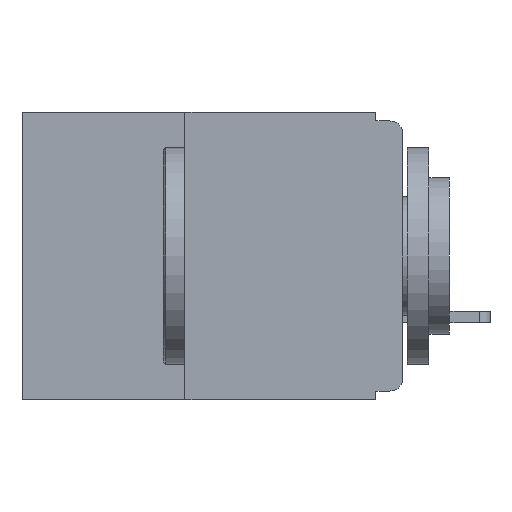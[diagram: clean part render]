
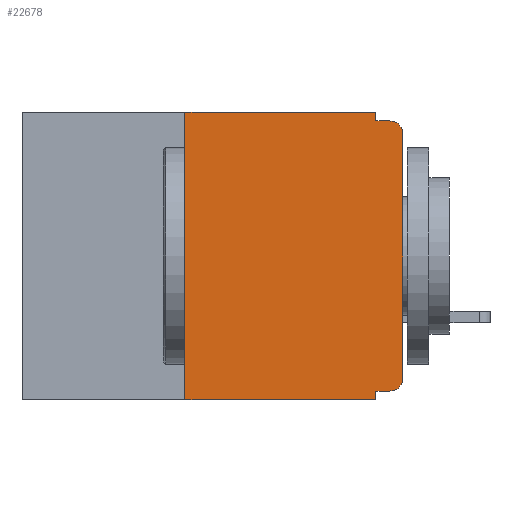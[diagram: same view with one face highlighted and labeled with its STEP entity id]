
A CAD part, left-side view. The second image highlights one B-rep face of the part: STEP entity #22678.
In plain terms, the highlighted planar face has unit normal (-1, 0, 0).
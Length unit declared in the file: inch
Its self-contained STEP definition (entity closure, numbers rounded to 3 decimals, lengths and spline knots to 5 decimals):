
#242 = VECTOR ( 'NONE', #19861, 39.37008 ) ;
#512 = VECTOR ( 'NONE', #14025, 39.37008 ) ;
#592 = CARTESIAN_POINT ( 'NONE',  ( 0., 0.25, -0.33 ) ) ;
#633 = DIRECTION ( 'NONE',  ( 0., 1., 0. ) ) ;
#688 = CARTESIAN_POINT ( 'NONE',  ( 0., 0., -0.305 ) ) ;
#809 = VERTEX_POINT ( 'NONE', #9481 ) ;
#838 = VERTEX_POINT ( 'NONE', #23414 ) ;
#1155 = DIRECTION ( 'NONE',  ( 0., 0., -1. ) ) ;
#1160 = CARTESIAN_POINT ( 'NONE',  ( 0., 0.031, -0.33 ) ) ;
#1646 = LINE ( 'NONE', #13008, #24526 ) ;
#2704 = CIRCLE ( 'NONE', #27872, 0.015 ) ;
#2880 = VECTOR ( 'NONE', #15317, 39.37008 ) ;
#3051 = DIRECTION ( 'NONE',  ( 0., 0., 1. ) ) ;
#3053 = EDGE_CURVE ( 'NONE', #838, #6656, #2704, .T. ) ;
#3118 = VECTOR ( 'NONE', #28104, 39.37008 ) ;
#3181 = ORIENTED_EDGE ( 'NONE', *, *, #4889, .F. ) ;
#4009 = EDGE_CURVE ( 'NONE', #23971, #8865, #12394, .T. ) ;
#4889 = EDGE_CURVE ( 'NONE', #809, #14808, #24730, .T. ) ;
#5514 = LINE ( 'NONE', #11851, #10742 ) ;
#5854 = AXIS2_PLACEMENT_3D ( 'NONE', #21785, #8538, #23991 ) ;
#6191 = ORIENTED_EDGE ( 'NONE', *, *, #4009, .F. ) ;
#6656 = VERTEX_POINT ( 'NONE', #688 ) ;
#7513 = EDGE_CURVE ( 'NONE', #24292, #8865, #10540, .T. ) ;
#7899 = VERTEX_POINT ( 'NONE', #18777 ) ;
#7981 = CARTESIAN_POINT ( 'NONE',  ( 0., 0., -0.025 ) ) ;
#8538 = DIRECTION ( 'NONE',  ( -1., 0., 0. ) ) ;
#8789 = LINE ( 'NONE', #28398, #2880 ) ;
#8865 = VERTEX_POINT ( 'NONE', #26378 ) ;
#9366 = EDGE_CURVE ( 'NONE', #12148, #14808, #26597, .T. ) ;
#9481 = CARTESIAN_POINT ( 'NONE',  ( 0., 0.031, -0.32 ) ) ;
#10540 = CIRCLE ( 'NONE', #5854, 0.015 ) ;
#10575 = CARTESIAN_POINT ( 'NONE',  ( 0., 0.437, -0.33 ) ) ;
#10742 = VECTOR ( 'NONE', #633, 39.37008 ) ;
#10921 = CARTESIAN_POINT ( 'NONE',  ( 0., 0.031, -0.01 ) ) ;
#11686 = PLANE ( 'NONE',  #23596 ) ;
#11851 = CARTESIAN_POINT ( 'NONE',  ( 0., 0., -0.32 ) ) ;
#12148 = VERTEX_POINT ( 'NONE', #592 ) ;
#12394 = LINE ( 'NONE', #13994, #512 ) ;
#13008 = CARTESIAN_POINT ( 'NONE',  ( 0., 0.25, -0.33 ) ) ;
#13031 = VECTOR ( 'NONE', #1155, 39.37008 ) ;
#13483 = EDGE_CURVE ( 'NONE', #838, #809, #5514, .T. ) ;
#13826 = EDGE_CURVE ( 'NONE', #12148, #7899, #1646, .T. ) ;
#13915 = DIRECTION ( 'NONE',  ( 0., 0., -1. ) ) ;
#13994 = CARTESIAN_POINT ( 'NONE',  ( 0., 0., -0.01 ) ) ;
#14025 = DIRECTION ( 'NONE',  ( 0., -1., 0. ) ) ;
#14808 = VERTEX_POINT ( 'NONE', #23632 ) ;
#15317 = DIRECTION ( 'NONE',  ( 0., 0., -1. ) ) ;
#15421 = LINE ( 'NONE', #16335, #16813 ) ;
#15725 = ORIENTED_EDGE ( 'NONE', *, *, #13483, .F. ) ;
#15883 = EDGE_CURVE ( 'NONE', #6656, #24292, #15421, .T. ) ;
#16335 = CARTESIAN_POINT ( 'NONE',  ( 0., 0., 0. ) ) ;
#16719 = FACE_OUTER_BOUND ( 'NONE', #17098, .T. ) ;
#16774 = EDGE_CURVE ( 'NONE', #25740, #23971, #8789, .T. ) ;
#16813 = VECTOR ( 'NONE', #3051, 39.37008 ) ;
#17098 = EDGE_LOOP ( 'NONE', ( #27651, #26703, #6191, #23794, #27467, #21826, #18689, #3181, #15725, #24739 ) ) ;
#18689 = ORIENTED_EDGE ( 'NONE', *, *, #9366, .T. ) ;
#18777 = CARTESIAN_POINT ( 'NONE',  ( 0., 0.25, 0. ) ) ;
#19635 = CARTESIAN_POINT ( 'NONE',  ( 0., 0.031, 0. ) ) ;
#19861 = DIRECTION ( 'NONE',  ( 0., -1., 0. ) ) ;
#21781 = DIRECTION ( 'NONE',  ( 0., 0., 1. ) ) ;
#21785 = CARTESIAN_POINT ( 'NONE',  ( 0., 0.015, -0.025 ) ) ;
#21826 = ORIENTED_EDGE ( 'NONE', *, *, #13826, .F. ) ;
#22678 = ADVANCED_FACE ( 'NONE', ( #16719 ), #11686, .F. ) ;
#23414 = CARTESIAN_POINT ( 'NONE',  ( 0., 0.015, -0.32 ) ) ;
#23596 = AXIS2_PLACEMENT_3D ( 'NONE', #24878, #27041, #13915 ) ;
#23632 = CARTESIAN_POINT ( 'NONE',  ( 0., 0.031, -0.33 ) ) ;
#23794 = ORIENTED_EDGE ( 'NONE', *, *, #16774, .F. ) ;
#23971 = VERTEX_POINT ( 'NONE', #10921 ) ;
#23991 = DIRECTION ( 'NONE',  ( 0., 0., -1. ) ) ;
#24292 = VERTEX_POINT ( 'NONE', #7981 ) ;
#24526 = VECTOR ( 'NONE', #21781, 39.37008 ) ;
#24537 = LINE ( 'NONE', #26337, #242 ) ;
#24730 = LINE ( 'NONE', #1160, #13031 ) ;
#24739 = ORIENTED_EDGE ( 'NONE', *, *, #3053, .T. ) ;
#24878 = CARTESIAN_POINT ( 'NONE',  ( 0., 0.437, 0. ) ) ;
#25147 = EDGE_CURVE ( 'NONE', #7899, #25740, #24537, .T. ) ;
#25740 = VERTEX_POINT ( 'NONE', #19635 ) ;
#26337 = CARTESIAN_POINT ( 'NONE',  ( 0., 0.437, 0. ) ) ;
#26378 = CARTESIAN_POINT ( 'NONE',  ( 0., 0.015, -0.01 ) ) ;
#26597 = LINE ( 'NONE', #10575, #3118 ) ;
#26703 = ORIENTED_EDGE ( 'NONE', *, *, #7513, .T. ) ;
#27041 = DIRECTION ( 'NONE',  ( 1., 0., 0. ) ) ;
#27467 = ORIENTED_EDGE ( 'NONE', *, *, #25147, .F. ) ;
#27651 = ORIENTED_EDGE ( 'NONE', *, *, #15883, .T. ) ;
#27872 = AXIS2_PLACEMENT_3D ( 'NONE', #28519, #28455, #28452 ) ;
#28104 = DIRECTION ( 'NONE',  ( 0., -1., 0. ) ) ;
#28398 = CARTESIAN_POINT ( 'NONE',  ( 0., 0.031, 0. ) ) ;
#28452 = DIRECTION ( 'NONE',  ( 0., 0., -1. ) ) ;
#28455 = DIRECTION ( 'NONE',  ( -1., 0., 0. ) ) ;
#28519 = CARTESIAN_POINT ( 'NONE',  ( 0., 0.015, -0.305 ) ) ;
